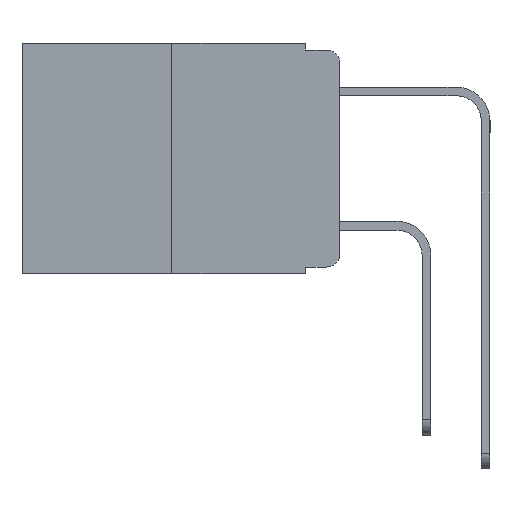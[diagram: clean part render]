
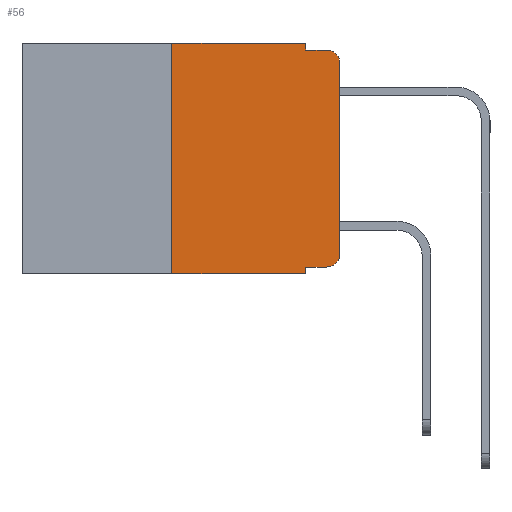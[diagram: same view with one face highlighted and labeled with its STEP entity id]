
A CAD part, left-side view. The second image highlights one B-rep face of the part: STEP entity #56.
In plain terms, the highlighted planar face has unit normal (-1, 0, 0).
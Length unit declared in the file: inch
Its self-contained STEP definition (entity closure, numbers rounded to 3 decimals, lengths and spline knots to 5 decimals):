
#56 = ADVANCED_FACE ( 'NONE', ( #13628 ), #6635, .F. ) ;
#173 = CARTESIAN_POINT ( 'NONE',  ( 0., 0.051, -0.333 ) ) ;
#302 = DIRECTION ( 'NONE',  ( 0., 0., -1. ) ) ;
#507 = CARTESIAN_POINT ( 'NONE',  ( 0., 0.051, -0.01 ) ) ;
#535 = DIRECTION ( 'NONE',  ( 0., -1., 0. ) ) ;
#865 = EDGE_LOOP ( 'NONE', ( #2971, #12499, #3390, #9967, #3800, #7270, #7669, #8048, #10952, #8421 ) ) ;
#1017 = DIRECTION ( 'NONE',  ( 0., -1., 0. ) ) ;
#1093 = EDGE_CURVE ( 'NONE', #13352, #1789, #5110, .T. ) ;
#1096 = EDGE_CURVE ( 'NONE', #6454, #7991, #8469, .T. ) ;
#1120 = DIRECTION ( 'NONE',  ( 0., 0., -1. ) ) ;
#1617 = CARTESIAN_POINT ( 'NONE',  ( 0., 0.473, 0. ) ) ;
#1789 = VERTEX_POINT ( 'NONE', #13428 ) ;
#2173 = DIRECTION ( 'NONE',  ( 0., 0., -1. ) ) ;
#2378 = CARTESIAN_POINT ( 'NONE',  ( 0., 0.051, 0. ) ) ;
#2965 = VECTOR ( 'NONE', #5363, 39.37008 ) ;
#2971 = ORIENTED_EDGE ( 'NONE', *, *, #7302, .T. ) ;
#3113 = VERTEX_POINT ( 'NONE', #5228 ) ;
#3181 = EDGE_CURVE ( 'NONE', #13352, #12671, #12823, .T. ) ;
#3390 = ORIENTED_EDGE ( 'NONE', *, *, #1096, .F. ) ;
#3800 = ORIENTED_EDGE ( 'NONE', *, *, #8842, .F. ) ;
#4188 = CARTESIAN_POINT ( 'NONE',  ( 0., 0.02, -0.313 ) ) ;
#4423 = LINE ( 'NONE', #4431, #10442 ) ;
#4431 = CARTESIAN_POINT ( 'NONE',  ( 0., 0., 0. ) ) ;
#4470 = AXIS2_PLACEMENT_3D ( 'NONE', #1617, #15303, #12467 ) ;
#4824 = CIRCLE ( 'NONE', #8103, 0.02 ) ;
#5110 = LINE ( 'NONE', #173, #11348 ) ;
#5119 = EDGE_CURVE ( 'NONE', #11986, #11775, #14431, .T. ) ;
#5121 = CARTESIAN_POINT ( 'NONE',  ( 0., 0.25, 0. ) ) ;
#5152 = EDGE_CURVE ( 'NONE', #14755, #6454, #5367, .T. ) ;
#5228 = CARTESIAN_POINT ( 'NONE',  ( 0., 0., -0.03 ) ) ;
#5307 = CARTESIAN_POINT ( 'NONE',  ( 0., 0.25, 0. ) ) ;
#5363 = DIRECTION ( 'NONE',  ( 0., -1., 0. ) ) ;
#5367 = LINE ( 'NONE', #11021, #10511 ) ;
#5529 = DIRECTION ( 'NONE',  ( 0., 0., -1. ) ) ;
#5843 = CIRCLE ( 'NONE', #13725, 0.02 ) ;
#6060 = LINE ( 'NONE', #12284, #2965 ) ;
#6445 = LINE ( 'NONE', #14178, #9621 ) ;
#6454 = VERTEX_POINT ( 'NONE', #7420 ) ;
#6561 = CARTESIAN_POINT ( 'NONE',  ( 0., 0.051, 0. ) ) ;
#6635 = PLANE ( 'NONE',  #4470 ) ;
#6998 = CARTESIAN_POINT ( 'NONE',  ( 0., 0.051, -0.333 ) ) ;
#7258 = EDGE_CURVE ( 'NONE', #3113, #7991, #4824, .T. ) ;
#7270 = ORIENTED_EDGE ( 'NONE', *, *, #5119, .F. ) ;
#7302 = EDGE_CURVE ( 'NONE', #13517, #3113, #4423, .T. ) ;
#7420 = CARTESIAN_POINT ( 'NONE',  ( 0., 0.051, -0.01 ) ) ;
#7499 = EDGE_CURVE ( 'NONE', #11986, #12671, #6445, .T. ) ;
#7588 = DIRECTION ( 'NONE',  ( 0., -1., 0. ) ) ;
#7669 = ORIENTED_EDGE ( 'NONE', *, *, #7499, .T. ) ;
#7673 = EDGE_CURVE ( 'NONE', #1789, #13517, #5843, .T. ) ;
#7991 = VERTEX_POINT ( 'NONE', #11001 ) ;
#8048 = ORIENTED_EDGE ( 'NONE', *, *, #3181, .F. ) ;
#8103 = AXIS2_PLACEMENT_3D ( 'NONE', #14731, #8232, #302 ) ;
#8232 = DIRECTION ( 'NONE',  ( -1., 0., 0. ) ) ;
#8403 = CARTESIAN_POINT ( 'NONE',  ( 0., 0., -0.313 ) ) ;
#8421 = ORIENTED_EDGE ( 'NONE', *, *, #7673, .T. ) ;
#8469 = LINE ( 'NONE', #507, #10991 ) ;
#8842 = EDGE_CURVE ( 'NONE', #11775, #14755, #6060, .T. ) ;
#9621 = VECTOR ( 'NONE', #7588, 39.37008 ) ;
#9862 = CARTESIAN_POINT ( 'NONE',  ( 0., 0.051, -0.343 ) ) ;
#9967 = ORIENTED_EDGE ( 'NONE', *, *, #5152, .F. ) ;
#10442 = VECTOR ( 'NONE', #14775, 39.37008 ) ;
#10511 = VECTOR ( 'NONE', #1120, 39.37008 ) ;
#10952 = ORIENTED_EDGE ( 'NONE', *, *, #1093, .T. ) ;
#10991 = VECTOR ( 'NONE', #535, 39.37008 ) ;
#11001 = CARTESIAN_POINT ( 'NONE',  ( 0., 0.02, -0.01 ) ) ;
#11021 = CARTESIAN_POINT ( 'NONE',  ( 0., 0.051, 0. ) ) ;
#11348 = VECTOR ( 'NONE', #1017, 39.37008 ) ;
#11775 = VERTEX_POINT ( 'NONE', #5307 ) ;
#11986 = VERTEX_POINT ( 'NONE', #13559 ) ;
#12284 = CARTESIAN_POINT ( 'NONE',  ( 0., 0.473, 0. ) ) ;
#12415 = DIRECTION ( 'NONE',  ( -1., 0., 0. ) ) ;
#12467 = DIRECTION ( 'NONE',  ( 0., 0., -1. ) ) ;
#12499 = ORIENTED_EDGE ( 'NONE', *, *, #7258, .T. ) ;
#12671 = VERTEX_POINT ( 'NONE', #9862 ) ;
#12823 = LINE ( 'NONE', #2378, #15284 ) ;
#13352 = VERTEX_POINT ( 'NONE', #6998 ) ;
#13428 = CARTESIAN_POINT ( 'NONE',  ( 0., 0.02, -0.333 ) ) ;
#13517 = VERTEX_POINT ( 'NONE', #8403 ) ;
#13559 = CARTESIAN_POINT ( 'NONE',  ( 0., 0.25, -0.343 ) ) ;
#13628 = FACE_OUTER_BOUND ( 'NONE', #865, .T. ) ;
#13725 = AXIS2_PLACEMENT_3D ( 'NONE', #4188, #12415, #5529 ) ;
#14103 = VECTOR ( 'NONE', #14267, 39.37008 ) ;
#14178 = CARTESIAN_POINT ( 'NONE',  ( 0., 0.473, -0.343 ) ) ;
#14267 = DIRECTION ( 'NONE',  ( 0., 0., 1. ) ) ;
#14431 = LINE ( 'NONE', #5121, #14103 ) ;
#14731 = CARTESIAN_POINT ( 'NONE',  ( 0., 0.02, -0.03 ) ) ;
#14755 = VERTEX_POINT ( 'NONE', #6561 ) ;
#14775 = DIRECTION ( 'NONE',  ( 0., 0., 1. ) ) ;
#15284 = VECTOR ( 'NONE', #2173, 39.37008 ) ;
#15303 = DIRECTION ( 'NONE',  ( 1., 0., 0. ) ) ;
